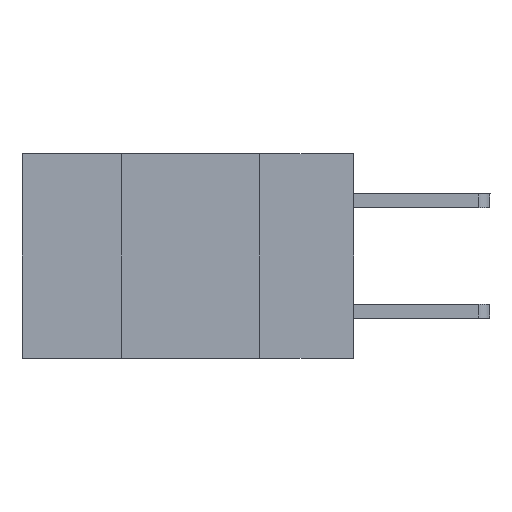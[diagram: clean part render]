
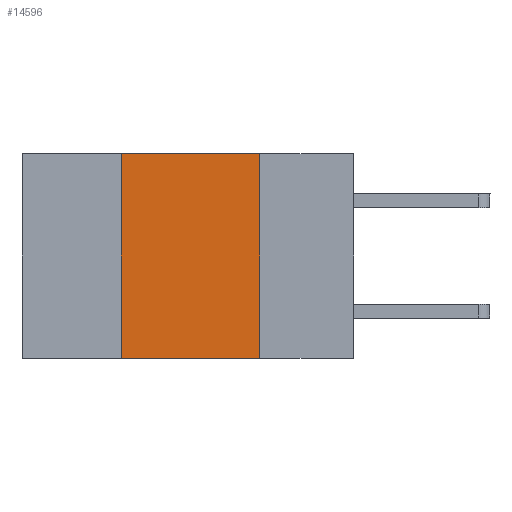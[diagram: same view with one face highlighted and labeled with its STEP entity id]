
A CAD part, left-side view. The second image highlights one B-rep face of the part: STEP entity #14596.
In plain terms, the highlighted planar face has unit normal (-1, 0, 0).
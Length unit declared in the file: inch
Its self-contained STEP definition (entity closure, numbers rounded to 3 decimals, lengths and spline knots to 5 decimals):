
#536 = ORIENTED_EDGE ( 'NONE', *, *, #4095, .F. ) ;
#977 = DIRECTION ( 'NONE',  ( 0., -1., 0. ) ) ;
#1138 = VECTOR ( 'NONE', #977, 39.37008 ) ;
#1336 = LINE ( 'NONE', #14047, #1138 ) ;
#1368 = AXIS2_PLACEMENT_3D ( 'NONE', #2477, #9716, #8544 ) ;
#1407 = CARTESIAN_POINT ( 'NONE',  ( 0., 0.42, -0.37 ) ) ;
#2477 = CARTESIAN_POINT ( 'NONE',  ( 0., 0.6, 0. ) ) ;
#3121 = VERTEX_POINT ( 'NONE', #13178 ) ;
#3660 = PLANE ( 'NONE',  #1368 ) ;
#4095 = EDGE_CURVE ( 'NONE', #10836, #3121, #9959, .T. ) ;
#4141 = CARTESIAN_POINT ( 'NONE',  ( 0., 0.42, 0. ) ) ;
#4190 = VECTOR ( 'NONE', #14494, 39.37008 ) ;
#4263 = ORIENTED_EDGE ( 'NONE', *, *, #9745, .T. ) ;
#4845 = ORIENTED_EDGE ( 'NONE', *, *, #8455, .F. ) ;
#4949 = LINE ( 'NONE', #14555, #4190 ) ;
#6427 = CARTESIAN_POINT ( 'NONE',  ( 0., 0.17, 0. ) ) ;
#7714 = EDGE_LOOP ( 'NONE', ( #536, #8810, #4845, #4263 ) ) ;
#8455 = EDGE_CURVE ( 'NONE', #15978, #14076, #9072, .T. ) ;
#8544 = DIRECTION ( 'NONE',  ( 0., 0., -1. ) ) ;
#8810 = ORIENTED_EDGE ( 'NONE', *, *, #10533, .F. ) ;
#8860 = DIRECTION ( 'NONE',  ( 0., 0., -1. ) ) ;
#8898 = CARTESIAN_POINT ( 'NONE',  ( 0., 0.17, 0. ) ) ;
#9072 = LINE ( 'NONE', #4141, #15144 ) ;
#9716 = DIRECTION ( 'NONE',  ( 1., 0., 0. ) ) ;
#9745 = EDGE_CURVE ( 'NONE', #15978, #3121, #1336, .T. ) ;
#9959 = LINE ( 'NONE', #6427, #15259 ) ;
#10521 = DIRECTION ( 'NONE',  ( 0., 0., 1. ) ) ;
#10533 = EDGE_CURVE ( 'NONE', #14076, #10836, #4949, .T. ) ;
#10836 = VERTEX_POINT ( 'NONE', #8898 ) ;
#12116 = FACE_OUTER_BOUND ( 'NONE', #7714, .T. ) ;
#13178 = CARTESIAN_POINT ( 'NONE',  ( 0., 0.17, -0.37 ) ) ;
#13450 = CARTESIAN_POINT ( 'NONE',  ( 0., 0.42, 0. ) ) ;
#14047 = CARTESIAN_POINT ( 'NONE',  ( 0., 0.6, -0.37 ) ) ;
#14076 = VERTEX_POINT ( 'NONE', #13450 ) ;
#14494 = DIRECTION ( 'NONE',  ( 0., -1., 0. ) ) ;
#14555 = CARTESIAN_POINT ( 'NONE',  ( 0., 0.6, 0. ) ) ;
#14596 = ADVANCED_FACE ( 'NONE', ( #12116 ), #3660, .F. ) ;
#15144 = VECTOR ( 'NONE', #10521, 39.37008 ) ;
#15259 = VECTOR ( 'NONE', #8860, 39.37008 ) ;
#15978 = VERTEX_POINT ( 'NONE', #1407 ) ;
